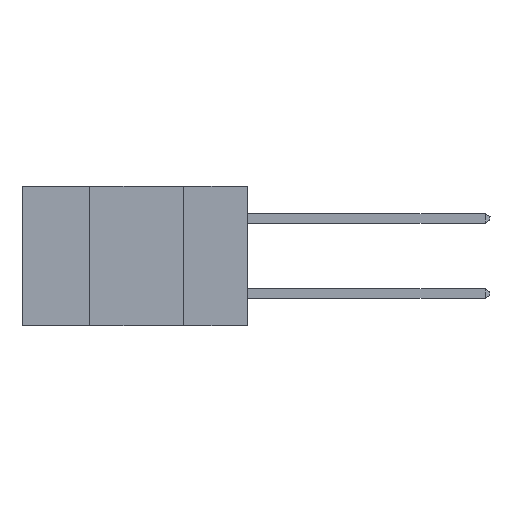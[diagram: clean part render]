
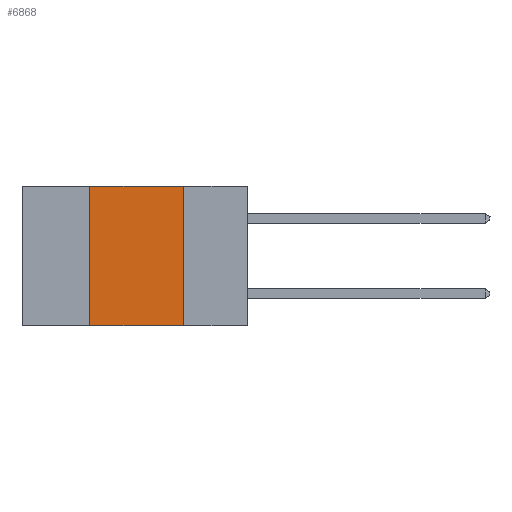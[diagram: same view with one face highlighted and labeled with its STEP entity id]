
A CAD part, left-side view. The second image highlights one B-rep face of the part: STEP entity #6868.
In plain terms, the highlighted planar face has unit normal (-1, 0, 0).
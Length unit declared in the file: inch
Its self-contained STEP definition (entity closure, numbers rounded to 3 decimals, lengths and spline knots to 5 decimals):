
#187 = CARTESIAN_POINT ( 'NONE',  ( 0., 0.6, -0.37 ) ) ;
#286 = CARTESIAN_POINT ( 'NONE',  ( 0., 0.6, 0. ) ) ;
#2693 = CARTESIAN_POINT ( 'NONE',  ( 0., 0.17, -0.37 ) ) ;
#2808 = VECTOR ( 'NONE', #6028, 39.37008 ) ;
#3505 = LINE ( 'NONE', #187, #16566 ) ;
#6028 = DIRECTION ( 'NONE',  ( 0., 0., 1. ) ) ;
#6124 = DIRECTION ( 'NONE',  ( 0., 0., -1. ) ) ;
#6163 = DIRECTION ( 'NONE',  ( 1., 0., 0. ) ) ;
#6211 = CARTESIAN_POINT ( 'NONE',  ( 0., 0.6, 0. ) ) ;
#6544 = PLANE ( 'NONE',  #8344 ) ;
#6868 = ADVANCED_FACE ( 'NONE', ( #22090 ), #6544, .F. ) ;
#6882 = ORIENTED_EDGE ( 'NONE', *, *, #10432, .F. ) ;
#7695 = ORIENTED_EDGE ( 'NONE', *, *, #22020, .T. ) ;
#8344 = AXIS2_PLACEMENT_3D ( 'NONE', #6211, #6163, #6124 ) ;
#9767 = LINE ( 'NONE', #11173, #2808 ) ;
#10432 = EDGE_CURVE ( 'NONE', #25978, #26394, #30156, .T. ) ;
#11173 = CARTESIAN_POINT ( 'NONE',  ( 0., 0.42, 0. ) ) ;
#12403 = CARTESIAN_POINT ( 'NONE',  ( 0., 0.42, 0. ) ) ;
#15810 = VECTOR ( 'NONE', #24572, 39.37008 ) ;
#16566 = VECTOR ( 'NONE', #21033, 39.37008 ) ;
#16874 = CARTESIAN_POINT ( 'NONE',  ( 0., 0.17, 0. ) ) ;
#18574 = LINE ( 'NONE', #286, #31276 ) ;
#19736 = EDGE_LOOP ( 'NONE', ( #6882, #24532, #32627, #7695 ) ) ;
#21033 = DIRECTION ( 'NONE',  ( 0., -1., 0. ) ) ;
#21131 = DIRECTION ( 'NONE',  ( 0., -1., 0. ) ) ;
#22020 = EDGE_CURVE ( 'NONE', #22758, #26394, #3505, .T. ) ;
#22090 = FACE_OUTER_BOUND ( 'NONE', #19736, .T. ) ;
#22758 = VERTEX_POINT ( 'NONE', #28957 ) ;
#24532 = ORIENTED_EDGE ( 'NONE', *, *, #27754, .F. ) ;
#24549 = CARTESIAN_POINT ( 'NONE',  ( 0., 0.17, 0. ) ) ;
#24572 = DIRECTION ( 'NONE',  ( 0., 0., -1. ) ) ;
#25845 = EDGE_CURVE ( 'NONE', #22758, #31350, #9767, .T. ) ;
#25978 = VERTEX_POINT ( 'NONE', #24549 ) ;
#26394 = VERTEX_POINT ( 'NONE', #2693 ) ;
#27754 = EDGE_CURVE ( 'NONE', #31350, #25978, #18574, .T. ) ;
#28957 = CARTESIAN_POINT ( 'NONE',  ( 0., 0.42, -0.37 ) ) ;
#30156 = LINE ( 'NONE', #16874, #15810 ) ;
#31276 = VECTOR ( 'NONE', #21131, 39.37008 ) ;
#31350 = VERTEX_POINT ( 'NONE', #12403 ) ;
#32627 = ORIENTED_EDGE ( 'NONE', *, *, #25845, .F. ) ;
